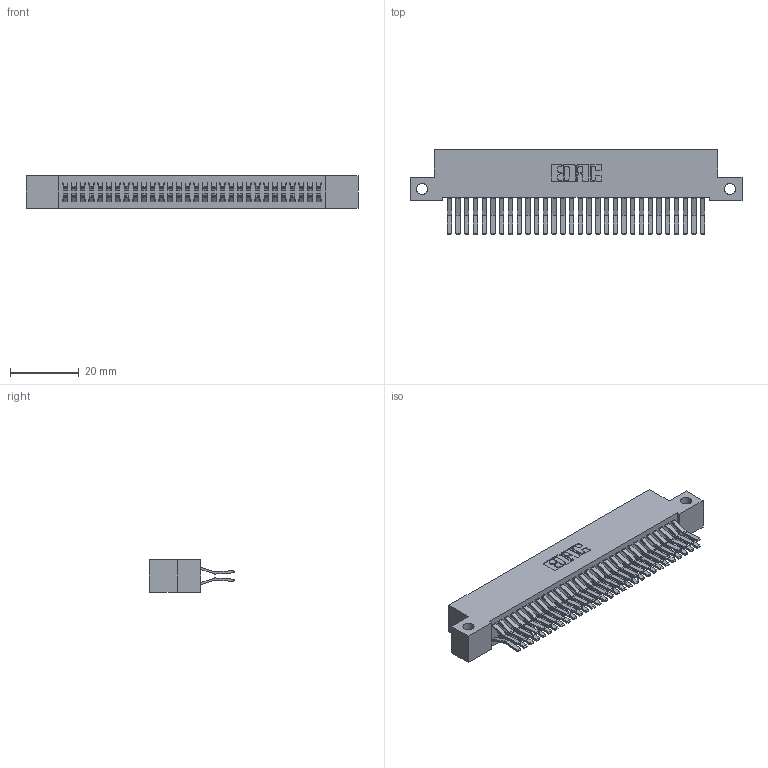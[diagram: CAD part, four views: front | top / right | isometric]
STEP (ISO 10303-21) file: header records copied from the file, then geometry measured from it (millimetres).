
FILE_DESCRIPTION (( 'STEP AP203' ), '1' );
FILE_NAME ('342-060-560-212.STEP', '2018-08-13T06:28:44', ( '' ), ( '' ), 'SwSTEP 2.0', 'SolidWorks 2016', '' );
FILE_SCHEMA (( 'CONFIG_CONTROL_DESIGN' ));
Length unit declared in the file: inch
Products named in the file (3): 342-060-560-212; 342 Part_Side Mount; 345-292-001_560 Tail
Assembly tree (61 placements, depth 2):
  342-060-560-212
    342 Part_Side Mount
    345-292-001_560 Tail  x60
Bounding box: 96.52 x 24.78 x 9.4 mm (x, y, z)
Volume: 8935.5 mm3; surface area: 15033.9 mm2
Topology: 61 solids, 61 shells, 3350 faces, 9959 edges, 6558 vertices
Faces by surface type: plane 2226, cylinder 1124
Entity records: 20811 total; most frequent: CARTESIAN_POINT 3462, ORIENTED_EDGE 3398, DIRECTION 2983, EDGE_CURVE 1699, VECTOR 1567, LINE 1567, VERTEX_POINT 1130, AXIS2_PLACEMENT_3D 708
